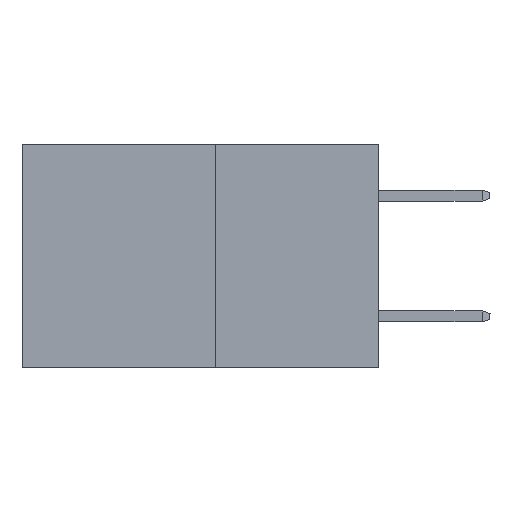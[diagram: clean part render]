
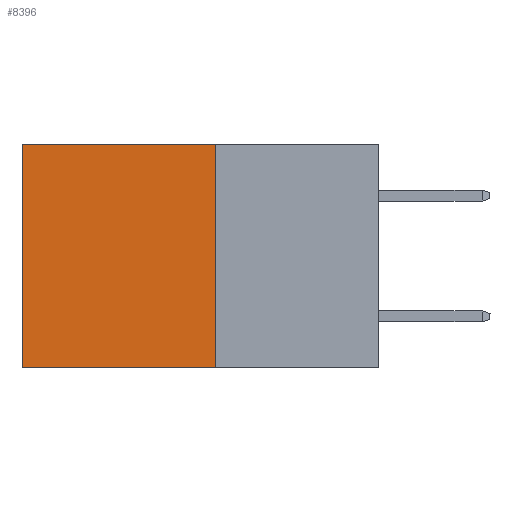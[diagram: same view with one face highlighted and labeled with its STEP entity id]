
A CAD part, left-side view. The second image highlights one B-rep face of the part: STEP entity #8396.
In plain terms, the highlighted planar face has unit normal (-1, 0, 0).
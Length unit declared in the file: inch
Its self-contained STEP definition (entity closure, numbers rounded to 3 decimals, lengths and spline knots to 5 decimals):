
#507 = CARTESIAN_POINT ( 'NONE',  ( 0.277, 0.27, 0. ) ) ;
#1066 = VERTEX_POINT ( 'NONE', #1144 ) ;
#1144 = CARTESIAN_POINT ( 'NONE',  ( 0.277, 0.59, 0. ) ) ;
#1479 = ORIENTED_EDGE ( 'NONE', *, *, #11530, .T. ) ;
#2110 = EDGE_LOOP ( 'NONE', ( #11016, #15435, #6979, #1479 ) ) ;
#2823 = DIRECTION ( 'NONE',  ( 0., 0., -1. ) ) ;
#3481 = LINE ( 'NONE', #5864, #6537 ) ;
#3918 = EDGE_CURVE ( 'NONE', #14486, #3988, #3481, .T. ) ;
#3963 = EDGE_CURVE ( 'NONE', #5134, #14486, #6118, .T. ) ;
#3988 = VERTEX_POINT ( 'NONE', #5961 ) ;
#4640 = CARTESIAN_POINT ( 'NONE',  ( 0.277, 0.27, -0.37 ) ) ;
#5134 = VERTEX_POINT ( 'NONE', #13656 ) ;
#5864 = CARTESIAN_POINT ( 'NONE',  ( 0.277, 0.27, -0.37 ) ) ;
#5894 = LINE ( 'NONE', #507, #12415 ) ;
#5961 = CARTESIAN_POINT ( 'NONE',  ( 0.277, 0.59, -0.37 ) ) ;
#6118 = LINE ( 'NONE', #9734, #16108 ) ;
#6537 = VECTOR ( 'NONE', #7193, 39.37008 ) ;
#6784 = VECTOR ( 'NONE', #2823, 39.37008 ) ;
#6979 = ORIENTED_EDGE ( 'NONE', *, *, #3963, .F. ) ;
#7193 = DIRECTION ( 'NONE',  ( 0., 1., 0. ) ) ;
#7264 = PLANE ( 'NONE',  #7293 ) ;
#7293 = AXIS2_PLACEMENT_3D ( 'NONE', #4640, #16351, #8564 ) ;
#8396 = ADVANCED_FACE ( 'NONE', ( #14110 ), #7264, .F. ) ;
#8564 = DIRECTION ( 'NONE',  ( 0., 0., -1. ) ) ;
#9734 = CARTESIAN_POINT ( 'NONE',  ( 0.277, 0.27, -0.37 ) ) ;
#9847 = DIRECTION ( 'NONE',  ( 0., 0., -1. ) ) ;
#10660 = LINE ( 'NONE', #11932, #6784 ) ;
#10928 = DIRECTION ( 'NONE',  ( 0., 1., 0. ) ) ;
#11016 = ORIENTED_EDGE ( 'NONE', *, *, #16252, .T. ) ;
#11530 = EDGE_CURVE ( 'NONE', #5134, #1066, #5894, .T. ) ;
#11932 = CARTESIAN_POINT ( 'NONE',  ( 0.277, 0.59, -0.37 ) ) ;
#12415 = VECTOR ( 'NONE', #10928, 39.37008 ) ;
#13656 = CARTESIAN_POINT ( 'NONE',  ( 0.277, 0.27, 0. ) ) ;
#14110 = FACE_OUTER_BOUND ( 'NONE', #2110, .T. ) ;
#14486 = VERTEX_POINT ( 'NONE', #14931 ) ;
#14931 = CARTESIAN_POINT ( 'NONE',  ( 0.277, 0.27, -0.37 ) ) ;
#15435 = ORIENTED_EDGE ( 'NONE', *, *, #3918, .F. ) ;
#16108 = VECTOR ( 'NONE', #9847, 39.37008 ) ;
#16252 = EDGE_CURVE ( 'NONE', #1066, #3988, #10660, .T. ) ;
#16351 = DIRECTION ( 'NONE',  ( 1., 0., 0. ) ) ;
